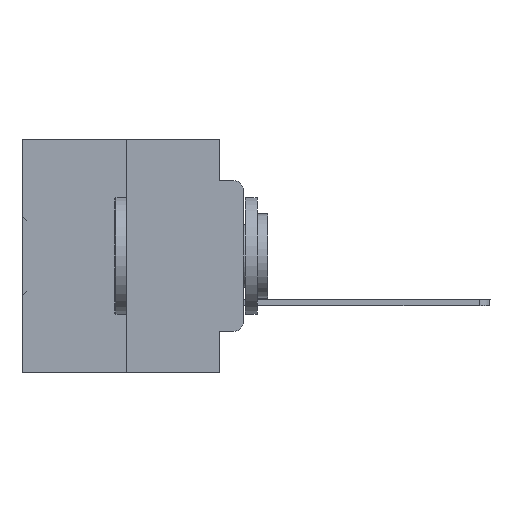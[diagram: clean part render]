
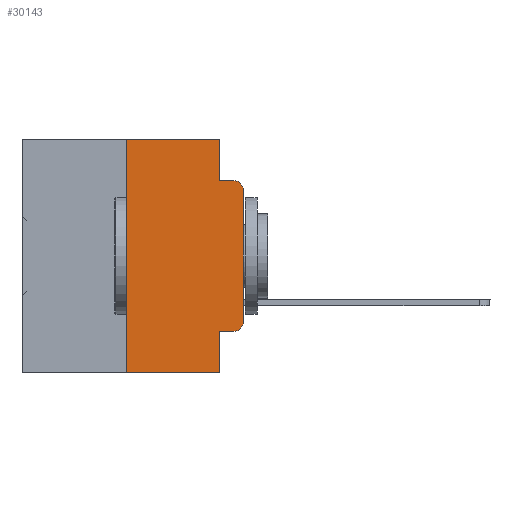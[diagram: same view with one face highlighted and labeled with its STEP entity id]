
A CAD part, left-side view. The second image highlights one B-rep face of the part: STEP entity #30143.
In plain terms, the highlighted planar face has unit normal (-1, 0, 0).
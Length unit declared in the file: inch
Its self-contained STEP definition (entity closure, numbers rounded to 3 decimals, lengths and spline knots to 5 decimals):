
#125 = VERTEX_POINT ( 'NONE', #14243 ) ;
#177 = LINE ( 'NONE', #17191, #1207 ) ;
#1207 = VECTOR ( 'NONE', #12044, 39.37008 ) ;
#1330 = EDGE_LOOP ( 'NONE', ( #29044, #23588, #20494, #5669, #14316, #27739, #19782, #32492, #13538, #28949 ) ) ;
#3064 = VERTEX_POINT ( 'NONE', #36604 ) ;
#3858 = LINE ( 'NONE', #13201, #26027 ) ;
#4045 = CARTESIAN_POINT ( 'NONE',  ( 0., 0.051, -0.5 ) ) ;
#4263 = CARTESIAN_POINT ( 'NONE',  ( 0., 0.473, 0. ) ) ;
#4731 = LINE ( 'NONE', #22333, #17411 ) ;
#5209 = DIRECTION ( 'NONE',  ( 0., -1., 0. ) ) ;
#5669 = ORIENTED_EDGE ( 'NONE', *, *, #15214, .F. ) ;
#6303 = EDGE_CURVE ( 'NONE', #3064, #25503, #12935, .T. ) ;
#6861 = EDGE_CURVE ( 'NONE', #23507, #125, #31218, .T. ) ;
#7248 = DIRECTION ( 'NONE',  ( 0., -1., 0. ) ) ;
#7597 = CARTESIAN_POINT ( 'NONE',  ( 0., 0.25, 0. ) ) ;
#8873 = EDGE_CURVE ( 'NONE', #11825, #18302, #22475, .T. ) ;
#9633 = VERTEX_POINT ( 'NONE', #13603 ) ;
#9638 = PLANE ( 'NONE',  #29291 ) ;
#9786 = DIRECTION ( 'NONE',  ( 0., 0., -1. ) ) ;
#9864 = VERTEX_POINT ( 'NONE', #13656 ) ;
#10530 = CARTESIAN_POINT ( 'NONE',  ( 0., 0.051, 0. ) ) ;
#11511 = LINE ( 'NONE', #26608, #18936 ) ;
#11825 = VERTEX_POINT ( 'NONE', #11883 ) ;
#11883 = CARTESIAN_POINT ( 'NONE',  ( 0., 0.02, -0.4115 ) ) ;
#12044 = DIRECTION ( 'NONE',  ( 0., -1., 0. ) ) ;
#12735 = AXIS2_PLACEMENT_3D ( 'NONE', #14419, #26076, #17447 ) ;
#12935 = LINE ( 'NONE', #33351, #32379 ) ;
#13074 = DIRECTION ( 'NONE',  ( 0., 0., -1. ) ) ;
#13170 = CARTESIAN_POINT ( 'NONE',  ( 0., 0., 0. ) ) ;
#13201 = CARTESIAN_POINT ( 'NONE',  ( 0., 0.051, 0. ) ) ;
#13368 = AXIS2_PLACEMENT_3D ( 'NONE', #15840, #24476, #36111 ) ;
#13538 = ORIENTED_EDGE ( 'NONE', *, *, #26232, .T. ) ;
#13603 = CARTESIAN_POINT ( 'NONE',  ( 0., 0., -0.1085 ) ) ;
#13656 = CARTESIAN_POINT ( 'NONE',  ( 0., 0.051, -0.4115 ) ) ;
#14243 = CARTESIAN_POINT ( 'NONE',  ( 0., 0.02, -0.0885 ) ) ;
#14316 = ORIENTED_EDGE ( 'NONE', *, *, #20326, .F. ) ;
#14419 = CARTESIAN_POINT ( 'NONE',  ( 0., 0.02, -0.3915 ) ) ;
#15214 = EDGE_CURVE ( 'NONE', #36104, #23507, #3858, .T. ) ;
#15840 = CARTESIAN_POINT ( 'NONE',  ( 0., 0.02, -0.1085 ) ) ;
#15844 = EDGE_CURVE ( 'NONE', #9864, #25503, #4731, .T. ) ;
#16197 = LINE ( 'NONE', #24816, #30248 ) ;
#16478 = CARTESIAN_POINT ( 'NONE',  ( 0., 0.051, -0.0885 ) ) ;
#17191 = CARTESIAN_POINT ( 'NONE',  ( 0., 0.473, 0. ) ) ;
#17411 = VECTOR ( 'NONE', #28610, 39.37008 ) ;
#17447 = DIRECTION ( 'NONE',  ( 0., 0., -1. ) ) ;
#18302 = VERTEX_POINT ( 'NONE', #35968 ) ;
#18771 = FACE_OUTER_BOUND ( 'NONE', #1330, .T. ) ;
#18814 = DIRECTION ( 'NONE',  ( 0., -1., 0. ) ) ;
#18936 = VECTOR ( 'NONE', #19899, 39.37008 ) ;
#19782 = ORIENTED_EDGE ( 'NONE', *, *, #6303, .T. ) ;
#19899 = DIRECTION ( 'NONE',  ( 0., 0., 1. ) ) ;
#20326 = EDGE_CURVE ( 'NONE', #32782, #36104, #177, .T. ) ;
#20494 = ORIENTED_EDGE ( 'NONE', *, *, #6861, .F. ) ;
#22333 = CARTESIAN_POINT ( 'NONE',  ( 0., 0.051, 0. ) ) ;
#22475 = CIRCLE ( 'NONE', #12735, 0.02 ) ;
#23507 = VERTEX_POINT ( 'NONE', #25725 ) ;
#23588 = ORIENTED_EDGE ( 'NONE', *, *, #29285, .T. ) ;
#24476 = DIRECTION ( 'NONE',  ( -1., 0., 0. ) ) ;
#24816 = CARTESIAN_POINT ( 'NONE',  ( 0., 0.051, -0.4115 ) ) ;
#25503 = VERTEX_POINT ( 'NONE', #4045 ) ;
#25725 = CARTESIAN_POINT ( 'NONE',  ( 0., 0.051, -0.0885 ) ) ;
#26027 = VECTOR ( 'NONE', #9786, 39.37008 ) ;
#26076 = DIRECTION ( 'NONE',  ( -1., 0., 0. ) ) ;
#26232 = EDGE_CURVE ( 'NONE', #9864, #11825, #16197, .T. ) ;
#26608 = CARTESIAN_POINT ( 'NONE',  ( 0., 0.25, 0. ) ) ;
#27589 = DIRECTION ( 'NONE',  ( 1., 0., 0. ) ) ;
#27643 = EDGE_CURVE ( 'NONE', #18302, #9633, #33410, .T. ) ;
#27739 = ORIENTED_EDGE ( 'NONE', *, *, #30381, .F. ) ;
#28610 = DIRECTION ( 'NONE',  ( 0., 0., -1. ) ) ;
#28949 = ORIENTED_EDGE ( 'NONE', *, *, #8873, .T. ) ;
#29044 = ORIENTED_EDGE ( 'NONE', *, *, #27643, .T. ) ;
#29285 = EDGE_CURVE ( 'NONE', #9633, #125, #29840, .T. ) ;
#29291 = AXIS2_PLACEMENT_3D ( 'NONE', #4263, #27589, #13074 ) ;
#29840 = CIRCLE ( 'NONE', #13368, 0.02 ) ;
#30143 = ADVANCED_FACE ( 'NONE', ( #18771 ), #9638, .F. ) ;
#30248 = VECTOR ( 'NONE', #7248, 39.37008 ) ;
#30381 = EDGE_CURVE ( 'NONE', #3064, #32782, #11511, .T. ) ;
#30561 = DIRECTION ( 'NONE',  ( 0., 0., 1. ) ) ;
#30612 = VECTOR ( 'NONE', #5209, 39.37008 ) ;
#31218 = LINE ( 'NONE', #16478, #30612 ) ;
#32379 = VECTOR ( 'NONE', #18814, 39.37008 ) ;
#32492 = ORIENTED_EDGE ( 'NONE', *, *, #15844, .F. ) ;
#32782 = VERTEX_POINT ( 'NONE', #7597 ) ;
#33351 = CARTESIAN_POINT ( 'NONE',  ( 0., 0.473, -0.5 ) ) ;
#33410 = LINE ( 'NONE', #13170, #35859 ) ;
#35859 = VECTOR ( 'NONE', #30561, 39.37008 ) ;
#35968 = CARTESIAN_POINT ( 'NONE',  ( 0., 0., -0.3915 ) ) ;
#36104 = VERTEX_POINT ( 'NONE', #10530 ) ;
#36111 = DIRECTION ( 'NONE',  ( 0., 0., -1. ) ) ;
#36604 = CARTESIAN_POINT ( 'NONE',  ( 0., 0.25, -0.5 ) ) ;
